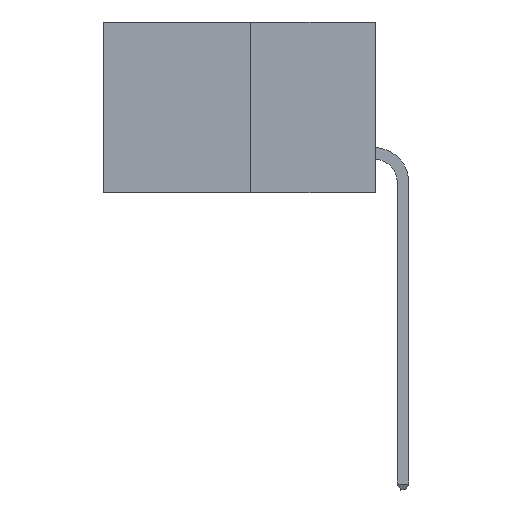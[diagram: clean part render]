
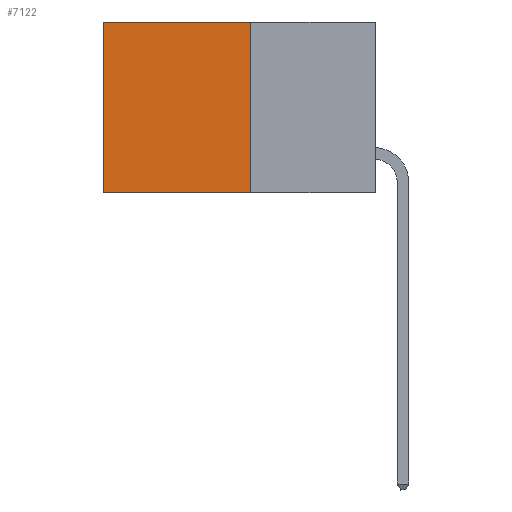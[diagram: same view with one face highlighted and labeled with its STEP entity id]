
A CAD part, left-side view. The second image highlights one B-rep face of the part: STEP entity #7122.
In plain terms, the highlighted planar face has unit normal (-1, 0, 0).
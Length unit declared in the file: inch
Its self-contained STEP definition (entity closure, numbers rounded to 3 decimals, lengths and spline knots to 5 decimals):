
#76 = CARTESIAN_POINT ( 'NONE',  ( 0.277, 0.27, 0. ) ) ;
#361 = ORIENTED_EDGE ( 'NONE', *, *, #14931, .T. ) ;
#972 = EDGE_LOOP ( 'NONE', ( #361, #13296, #1680, #5166 ) ) ;
#1680 = ORIENTED_EDGE ( 'NONE', *, *, #13840, .F. ) ;
#1934 = DIRECTION ( 'NONE',  ( 0., 0., -1. ) ) ;
#2410 = DIRECTION ( 'NONE',  ( 0., 1., 0. ) ) ;
#2760 = LINE ( 'NONE', #16683, #3220 ) ;
#3220 = VECTOR ( 'NONE', #2410, 39.37008 ) ;
#3938 = DIRECTION ( 'NONE',  ( 0., 0., -1. ) ) ;
#4984 = VERTEX_POINT ( 'NONE', #5938 ) ;
#5166 = ORIENTED_EDGE ( 'NONE', *, *, #11736, .T. ) ;
#5213 = DIRECTION ( 'NONE',  ( 1., 0., 0. ) ) ;
#5335 = LINE ( 'NONE', #15109, #12514 ) ;
#5938 = CARTESIAN_POINT ( 'NONE',  ( 0.277, 0.27, -0.37 ) ) ;
#6346 = CARTESIAN_POINT ( 'NONE',  ( 0.277, 0.59, -0.37 ) ) ;
#6954 = VERTEX_POINT ( 'NONE', #6346 ) ;
#7122 = ADVANCED_FACE ( 'NONE', ( #9314 ), #9546, .F. ) ;
#7337 = DIRECTION ( 'NONE',  ( 0., 1., 0. ) ) ;
#7894 = AXIS2_PLACEMENT_3D ( 'NONE', #13787, #5213, #15190 ) ;
#9314 = FACE_OUTER_BOUND ( 'NONE', #972, .T. ) ;
#9546 = PLANE ( 'NONE',  #7894 ) ;
#10407 = VECTOR ( 'NONE', #7337, 39.37008 ) ;
#10867 = LINE ( 'NONE', #17172, #10407 ) ;
#11022 = VECTOR ( 'NONE', #3938, 39.37008 ) ;
#11233 = VERTEX_POINT ( 'NONE', #16110 ) ;
#11736 = EDGE_CURVE ( 'NONE', #11750, #11233, #10867, .T. ) ;
#11750 = VERTEX_POINT ( 'NONE', #76 ) ;
#12514 = VECTOR ( 'NONE', #1934, 39.37008 ) ;
#13296 = ORIENTED_EDGE ( 'NONE', *, *, #15632, .F. ) ;
#13787 = CARTESIAN_POINT ( 'NONE',  ( 0.277, 0.27, -0.37 ) ) ;
#13840 = EDGE_CURVE ( 'NONE', #11750, #4984, #18014, .T. ) ;
#14931 = EDGE_CURVE ( 'NONE', #11233, #6954, #5335, .T. ) ;
#15109 = CARTESIAN_POINT ( 'NONE',  ( 0.277, 0.59, -0.37 ) ) ;
#15190 = DIRECTION ( 'NONE',  ( 0., 0., -1. ) ) ;
#15632 = EDGE_CURVE ( 'NONE', #4984, #6954, #2760, .T. ) ;
#16110 = CARTESIAN_POINT ( 'NONE',  ( 0.277, 0.59, 0. ) ) ;
#16680 = CARTESIAN_POINT ( 'NONE',  ( 0.277, 0.27, -0.37 ) ) ;
#16683 = CARTESIAN_POINT ( 'NONE',  ( 0.277, 0.27, -0.37 ) ) ;
#17172 = CARTESIAN_POINT ( 'NONE',  ( 0.277, 0.27, 0. ) ) ;
#18014 = LINE ( 'NONE', #16680, #11022 ) ;
